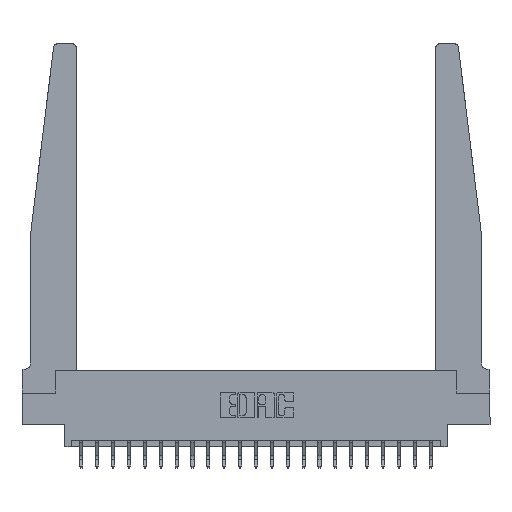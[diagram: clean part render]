
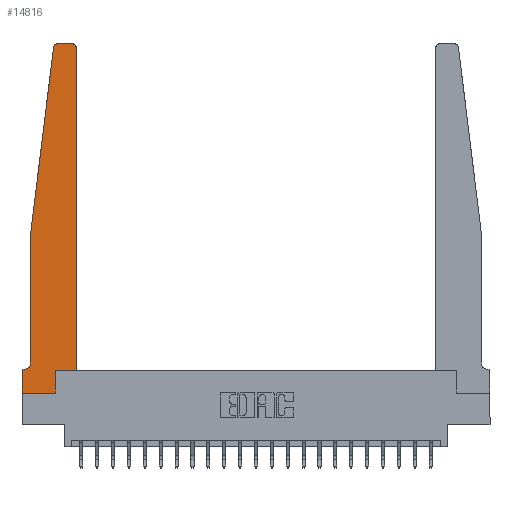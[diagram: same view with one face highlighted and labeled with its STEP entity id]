
A CAD part, top view. The second image highlights one B-rep face of the part: STEP entity #14816.
In plain terms, the highlighted planar face has unit normal (0, 0, 1).
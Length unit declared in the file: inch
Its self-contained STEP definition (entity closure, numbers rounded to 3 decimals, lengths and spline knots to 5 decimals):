
#60 = VERTEX_POINT ( 'NONE', #20228 ) ;
#99 = EDGE_CURVE ( 'NONE', #5702, #19435, #9896, .T. ) ;
#117 = CARTESIAN_POINT ( 'NONE',  ( 0.395, 2.72, 0.37 ) ) ;
#417 = DIRECTION ( 'NONE',  ( 1., 0., 0. ) ) ;
#725 = VECTOR ( 'NONE', #21835, 39.37008 ) ;
#1336 = VERTEX_POINT ( 'NONE', #12097 ) ;
#1341 = EDGE_CURVE ( 'NONE', #12899, #8633, #19262, .T. ) ;
#2088 = EDGE_CURVE ( 'NONE', #1336, #5702, #6256, .T. ) ;
#2191 = EDGE_CURVE ( 'NONE', #14108, #2327, #16894, .T. ) ;
#2327 = VERTEX_POINT ( 'NONE', #4856 ) ;
#2593 = CARTESIAN_POINT ( 'NONE',  ( 0., 0.1875, 0.37 ) ) ;
#2815 = FACE_OUTER_BOUND ( 'NONE', #13615, .T. ) ;
#2964 = EDGE_CURVE ( 'NONE', #60, #16100, #19781, .T. ) ;
#3769 = CIRCLE ( 'NONE', #15343, 0.03 ) ;
#3871 = AXIS2_PLACEMENT_3D ( 'NONE', #13809, #19089, #8758 ) ;
#3916 = VERTEX_POINT ( 'NONE', #14830 ) ;
#4025 = CARTESIAN_POINT ( 'NONE',  ( 0.425, 0.18, 0.37 ) ) ;
#4283 = VERTEX_POINT ( 'NONE', #11299 ) ;
#4342 = DIRECTION ( 'NONE',  ( 0., 0., -1. ) ) ;
#4632 = CARTESIAN_POINT ( 'NONE',  ( 0., 0., 0.37 ) ) ;
#4856 = CARTESIAN_POINT ( 'NONE',  ( 0., 0., 0.37 ) ) ;
#5171 = AXIS2_PLACEMENT_3D ( 'NONE', #2593, #17213, #11713 ) ;
#5218 = CARTESIAN_POINT ( 'NONE',  ( 0.065, 1.25, 0.37 ) ) ;
#5279 = DIRECTION ( 'NONE',  ( 0., 0., 1. ) ) ;
#5500 = EDGE_CURVE ( 'NONE', #2327, #4283, #13293, .T. ) ;
#5702 = VERTEX_POINT ( 'NONE', #8593 ) ;
#6256 = LINE ( 'NONE', #4025, #22410 ) ;
#6396 = EDGE_CURVE ( 'NONE', #4283, #1336, #15931, .T. ) ;
#6816 = EDGE_CURVE ( 'NONE', #19435, #60, #3769, .T. ) ;
#6825 = ORIENTED_EDGE ( 'NONE', *, *, #6396, .T. ) ;
#6904 = ORIENTED_EDGE ( 'NONE', *, *, #99, .T. ) ;
#7194 = VECTOR ( 'NONE', #19472, 39.37008 ) ;
#7286 = EDGE_CURVE ( 'NONE', #8633, #12292, #19754, .T. ) ;
#7317 = ORIENTED_EDGE ( 'NONE', *, *, #6816, .T. ) ;
#8065 = ORIENTED_EDGE ( 'NONE', *, *, #8996, .T. ) ;
#8363 = DIRECTION ( 'NONE',  ( 0., 1., 0. ) ) ;
#8587 = VECTOR ( 'NONE', #20211, 39.37008 ) ;
#8593 = CARTESIAN_POINT ( 'NONE',  ( 0.425, 0.18, 0.37 ) ) ;
#8633 = VERTEX_POINT ( 'NONE', #18052 ) ;
#8714 = DIRECTION ( 'NONE',  ( -0.122, -0.992, 0. ) ) ;
#8758 = DIRECTION ( 'NONE',  ( 1., 0., 0. ) ) ;
#8858 = ORIENTED_EDGE ( 'NONE', *, *, #2088, .T. ) ;
#8987 = ORIENTED_EDGE ( 'NONE', *, *, #2964, .T. ) ;
#8996 = EDGE_CURVE ( 'NONE', #16100, #12899, #13943, .T. ) ;
#9024 = CIRCLE ( 'NONE', #15769, 0.05 ) ;
#9029 = CARTESIAN_POINT ( 'NONE',  ( 0.2605, 0.18, 0.37 ) ) ;
#9896 = LINE ( 'NONE', #15513, #20759 ) ;
#10066 = PLANE ( 'NONE',  #5171 ) ;
#10833 = CARTESIAN_POINT ( 'NONE',  ( 0.065, 1.25, 0.37 ) ) ;
#11155 = ORIENTED_EDGE ( 'NONE', *, *, #2191, .T. ) ;
#11197 = VECTOR ( 'NONE', #12505, 39.37008 ) ;
#11299 = CARTESIAN_POINT ( 'NONE',  ( 0.2605, 0., 0.37 ) ) ;
#11336 = EDGE_CURVE ( 'NONE', #3916, #14108, #13054, .T. ) ;
#11469 = DIRECTION ( 'NONE',  ( -1., 0., 0. ) ) ;
#11506 = CARTESIAN_POINT ( 'NONE',  ( 0.425, 2.72, 0.37 ) ) ;
#11713 = DIRECTION ( 'NONE',  ( 1., 0., 0. ) ) ;
#12097 = CARTESIAN_POINT ( 'NONE',  ( 0.2605, 0.18, 0.37 ) ) ;
#12292 = VERTEX_POINT ( 'NONE', #19346 ) ;
#12505 = DIRECTION ( 'NONE',  ( -1., 0., 0. ) ) ;
#12756 = VECTOR ( 'NONE', #17643, 39.37008 ) ;
#12899 = VERTEX_POINT ( 'NONE', #15167 ) ;
#13054 = LINE ( 'NONE', #21846, #8587 ) ;
#13135 = CARTESIAN_POINT ( 'NONE',  ( 0.015, 0.2375, 0.37 ) ) ;
#13293 = LINE ( 'NONE', #4632, #20491 ) ;
#13615 = EDGE_LOOP ( 'NONE', ( #8987, #8065, #19161, #15753, #21348, #17533, #11155, #16848, #6825, #8858, #6904, #7317 ) ) ;
#13809 = CARTESIAN_POINT ( 'NONE',  ( 0.27653, 2.72, 0.37 ) ) ;
#13943 = CIRCLE ( 'NONE', #3871, 0.03 ) ;
#14108 = VERTEX_POINT ( 'NONE', #18835 ) ;
#14816 = ADVANCED_FACE ( 'NONE', ( #2815 ), #10066, .T. ) ;
#14830 = CARTESIAN_POINT ( 'NONE',  ( 0.015, 0.1875, 0.37 ) ) ;
#15167 = CARTESIAN_POINT ( 'NONE',  ( 0.24675, 2.72367, 0.37 ) ) ;
#15343 = AXIS2_PLACEMENT_3D ( 'NONE', #117, #5279, #22945 ) ;
#15513 = CARTESIAN_POINT ( 'NONE',  ( 0.425, 0.18, 0.37 ) ) ;
#15753 = ORIENTED_EDGE ( 'NONE', *, *, #7286, .T. ) ;
#15769 = AXIS2_PLACEMENT_3D ( 'NONE', #13135, #4342, #11469 ) ;
#15931 = LINE ( 'NONE', #9029, #7194 ) ;
#16100 = VERTEX_POINT ( 'NONE', #22287 ) ;
#16848 = ORIENTED_EDGE ( 'NONE', *, *, #5500, .T. ) ;
#16894 = LINE ( 'NONE', #18191, #725 ) ;
#17213 = DIRECTION ( 'NONE',  ( 0., 0., 1. ) ) ;
#17533 = ORIENTED_EDGE ( 'NONE', *, *, #11336, .T. ) ;
#17579 = EDGE_CURVE ( 'NONE', #12292, #3916, #9024, .T. ) ;
#17643 = DIRECTION ( 'NONE',  ( 0., -1., 0. ) ) ;
#18052 = CARTESIAN_POINT ( 'NONE',  ( 0.065, 1.25, 0.37 ) ) ;
#18191 = CARTESIAN_POINT ( 'NONE',  ( 0., 0., 0.37 ) ) ;
#18835 = CARTESIAN_POINT ( 'NONE',  ( 0., 0.1875, 0.37 ) ) ;
#19089 = DIRECTION ( 'NONE',  ( 0., 0., 1. ) ) ;
#19161 = ORIENTED_EDGE ( 'NONE', *, *, #1341, .T. ) ;
#19248 = VECTOR ( 'NONE', #8714, 39.37008 ) ;
#19262 = LINE ( 'NONE', #5218, #19248 ) ;
#19346 = CARTESIAN_POINT ( 'NONE',  ( 0.065, 0.2375, 0.37 ) ) ;
#19435 = VERTEX_POINT ( 'NONE', #11506 ) ;
#19472 = DIRECTION ( 'NONE',  ( 0., 1., 0. ) ) ;
#19754 = LINE ( 'NONE', #10833, #12756 ) ;
#19781 = LINE ( 'NONE', #21440, #11197 ) ;
#20211 = DIRECTION ( 'NONE',  ( -1., 0., 0. ) ) ;
#20228 = CARTESIAN_POINT ( 'NONE',  ( 0.395, 2.75, 0.37 ) ) ;
#20491 = VECTOR ( 'NONE', #21966, 39.37008 ) ;
#20759 = VECTOR ( 'NONE', #8363, 39.37008 ) ;
#21348 = ORIENTED_EDGE ( 'NONE', *, *, #17579, .T. ) ;
#21440 = CARTESIAN_POINT ( 'NONE',  ( 0.25, 2.75, 0.37 ) ) ;
#21835 = DIRECTION ( 'NONE',  ( 0., -1., 0. ) ) ;
#21846 = CARTESIAN_POINT ( 'NONE',  ( 0.065, 0.1875, 0.37 ) ) ;
#21966 = DIRECTION ( 'NONE',  ( 1., 0., 0. ) ) ;
#22287 = CARTESIAN_POINT ( 'NONE',  ( 0.27653, 2.75, 0.37 ) ) ;
#22410 = VECTOR ( 'NONE', #417, 39.37008 ) ;
#22945 = DIRECTION ( 'NONE',  ( 1., 0., 0. ) ) ;
